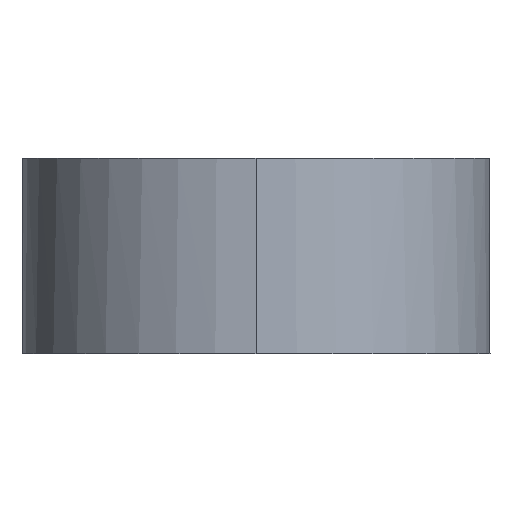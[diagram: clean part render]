
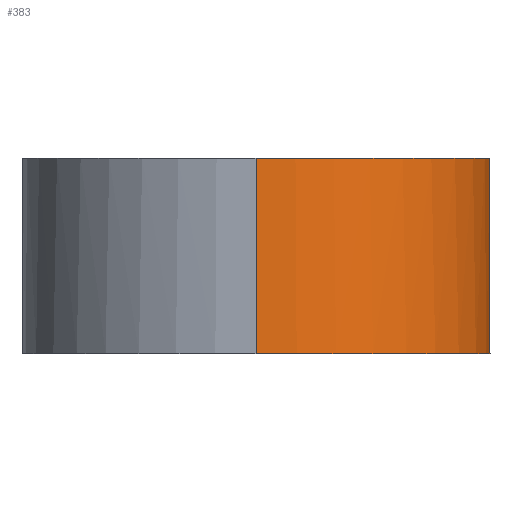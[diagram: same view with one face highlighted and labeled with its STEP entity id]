
A CAD part, left-side view. The second image highlights one B-rep face of the part: STEP entity #383.
In plain terms, the highlighted cylindrical face has radius 6 mm (diameter 12 mm), a partial arc.
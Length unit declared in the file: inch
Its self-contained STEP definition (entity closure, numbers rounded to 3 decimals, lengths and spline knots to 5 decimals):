
#2 = DIRECTION ( 'NONE',  ( -1., 0., 0. ) ) ;
#10 = DIRECTION ( 'NONE',  ( 0., 0., -1. ) ) ;
#26 = ORIENTED_EDGE ( 'NONE', *, *, #509, .T. ) ;
#46 = CARTESIAN_POINT ( 'NONE',  ( -4.61969, -0.57034, -2.75591 ) ) ;
#64 = LINE ( 'NONE', #812, #80 ) ;
#68 = VERTEX_POINT ( 'NONE', #394 ) ;
#72 = VERTEX_POINT ( 'NONE', #46 ) ;
#80 = VECTOR ( 'NONE', #357, 39.37008 ) ;
#82 = CARTESIAN_POINT ( 'NONE',  ( -4.62843, -0.58759, -2.76483 ) ) ;
#123 = VECTOR ( 'NONE', #10, 39.37008 ) ;
#132 = CARTESIAN_POINT ( 'NONE',  ( -4.62199, -0.57535, -2.75591 ) ) ;
#153 = CIRCLE ( 'NONE', #245, 0.23622 ) ;
#157 = FACE_OUTER_BOUND ( 'NONE', #233, .T. ) ;
#170 = CARTESIAN_POINT ( 'NONE',  ( -5.07065, -0.47191, -2.75591 ) ) ;
#219 = DIRECTION ( 'NONE',  ( 0., 0., -1. ) ) ;
#230 = B_SPLINE_CURVE_WITH_KNOTS ( 'NONE', 3,
 ( #351, #274, #82, #586, #132, #672 ),
 .UNSPECIFIED., .F., .F.,
 ( 4, 2, 4 ),
 ( 0., 0.00041, 0.00083 ),
 .UNSPECIFIED. ) ;
#233 = EDGE_LOOP ( 'NONE', ( #568, #237, #651, #428, #26 ) ) ;
#237 = ORIENTED_EDGE ( 'NONE', *, *, #718, .T. ) ;
#245 = AXIS2_PLACEMENT_3D ( 'NONE', #367, #219, #768 ) ;
#271 = AXIS2_PLACEMENT_3D ( 'NONE', #353, #866, #440 ) ;
#274 = CARTESIAN_POINT ( 'NONE',  ( -4.62986, -0.59002, -2.77006 ) ) ;
#278 = CARTESIAN_POINT ( 'NONE',  ( -4.83443, -0.47191, -2.75591 ) ) ;
#318 = VERTEX_POINT ( 'NONE', #170 ) ;
#336 = DIRECTION ( 'NONE',  ( 0., 0., -1. ) ) ;
#342 = CARTESIAN_POINT ( 'NONE',  ( -4.62986, -0.59002, -2.75591 ) ) ;
#351 = CARTESIAN_POINT ( 'NONE',  ( -4.62986, -0.59002, -2.77559 ) ) ;
#353 = CARTESIAN_POINT ( 'NONE',  ( -4.83443, -0.47191, -2.95276 ) ) ;
#357 = DIRECTION ( 'NONE',  ( 0., 0., -1. ) ) ;
#367 = CARTESIAN_POINT ( 'NONE',  ( -4.83443, -0.47191, -2.75591 ) ) ;
#383 = ADVANCED_FACE ( 'NONE', ( #157 ), #540, .T. ) ;
#394 = CARTESIAN_POINT ( 'NONE',  ( -5.07065, -0.47191, -2.95276 ) ) ;
#428 = ORIENTED_EDGE ( 'NONE', *, *, #479, .F. ) ;
#440 = DIRECTION ( 'NONE',  ( -1., 0., 0. ) ) ;
#446 = AXIS2_PLACEMENT_3D ( 'NONE', #278, #336, #2 ) ;
#479 = EDGE_CURVE ( 'NONE', #676, #557, #727, .T. ) ;
#509 = EDGE_CURVE ( 'NONE', #676, #72, #230, .T. ) ;
#540 = CYLINDRICAL_SURFACE ( 'NONE', #446, 0.23622 ) ;
#557 = VERTEX_POINT ( 'NONE', #758 ) ;
#568 = ORIENTED_EDGE ( 'NONE', *, *, #764, .T. ) ;
#586 = CARTESIAN_POINT ( 'NONE',  ( -4.62446, -0.58021, -2.75782 ) ) ;
#651 = ORIENTED_EDGE ( 'NONE', *, *, #712, .F. ) ;
#659 = CARTESIAN_POINT ( 'NONE',  ( -4.62986, -0.59002, -2.77559 ) ) ;
#672 = CARTESIAN_POINT ( 'NONE',  ( -4.61969, -0.57034, -2.75591 ) ) ;
#676 = VERTEX_POINT ( 'NONE', #659 ) ;
#712 = EDGE_CURVE ( 'NONE', #557, #68, #845, .T. ) ;
#718 = EDGE_CURVE ( 'NONE', #318, #68, #64, .T. ) ;
#727 = LINE ( 'NONE', #342, #123 ) ;
#758 = CARTESIAN_POINT ( 'NONE',  ( -4.62986, -0.59002, -2.95276 ) ) ;
#764 = EDGE_CURVE ( 'NONE', #72, #318, #153, .T. ) ;
#768 = DIRECTION ( 'NONE',  ( -1., 0., 0. ) ) ;
#812 = CARTESIAN_POINT ( 'NONE',  ( -5.07065, -0.47191, -2.75591 ) ) ;
#845 = CIRCLE ( 'NONE', #271, 0.23622 ) ;
#866 = DIRECTION ( 'NONE',  ( 0., 0., -1. ) ) ;
